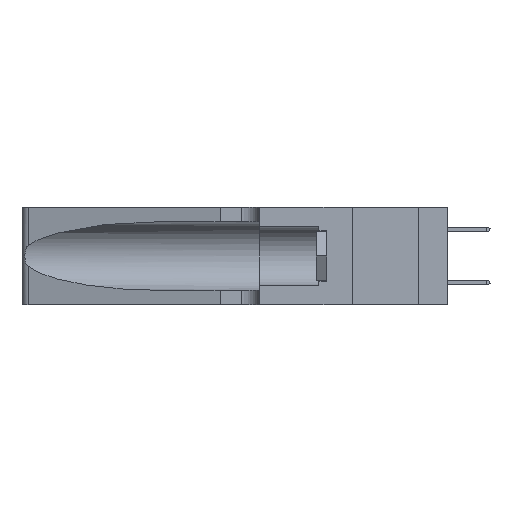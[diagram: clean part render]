
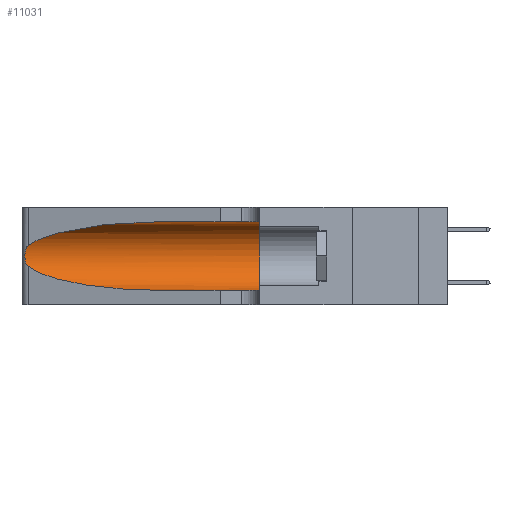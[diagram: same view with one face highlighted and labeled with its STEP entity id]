
A CAD part, left-side view. The second image highlights one B-rep face of the part: STEP entity #11031.
In plain terms, the highlighted cylindrical face has radius 3.308 mm (diameter 6.617 mm), a partial arc.
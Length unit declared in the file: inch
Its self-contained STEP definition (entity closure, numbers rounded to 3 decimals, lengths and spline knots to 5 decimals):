
#57 = CARTESIAN_POINT ( 'NONE',  ( 0.25487, 1.22718, 0.22369 ) ) ;
#100 = CARTESIAN_POINT ( 'NONE',  ( 0.1305, 0.72297, 0.31525 ) ) ;
#926 = CARTESIAN_POINT ( 'NONE',  ( 0.25487, 1.22718, 0.14631 ) ) ;
#1416 = EDGE_CURVE ( 'NONE', #9132, #16972, #7508, .T. ) ;
#1848 = CARTESIAN_POINT ( 'NONE',  ( 0.1305, 0.72297, 0.05475 ) ) ;
#1862 = ORIENTED_EDGE ( 'NONE', *, *, #10962, .T. ) ;
#2369 = CARTESIAN_POINT ( 'NONE',  ( 0.25487, 1.22718, 0.14631 ) ) ;
#2389 = CARTESIAN_POINT ( 'NONE',  ( 0.25639, 1.23184, 0.21858 ) ) ;
#2812 = ORIENTED_EDGE ( 'NONE', *, *, #8728, .F. ) ;
#2948 = CARTESIAN_POINT ( 'NONE',  ( 0.1305, 0.72297, 0.05475 ) ) ;
#3871 = CARTESIAN_POINT ( 'NONE',  ( 0.25854, 1.2359, 0.20912 ) ) ;
#4096 = EDGE_CURVE ( 'NONE', #6751, #18009, #15461, .T. ) ;
#4334 = LINE ( 'NONE', #5383, #11875 ) ;
#4336 = CARTESIAN_POINT ( 'NONE',  ( 0.2373, 1.15595, 0.08982 ) ) ;
#4714 = EDGE_CURVE ( 'NONE', #7164, #16972, #7858, .T. ) ;
#5213 = CARTESIAN_POINT ( 'NONE',  ( 0.1305, 0.72297, 0.31525 ) ) ;
#5281 = DIRECTION ( 'NONE',  ( 0., 1., 0. ) ) ;
#5329 = CARTESIAN_POINT ( 'NONE',  ( 0.26075, 1.23896, 0.19203 ) ) ;
#5383 = CARTESIAN_POINT ( 'NONE',  ( 0.1305, 1.61858, 0.31525 ) ) ;
#6339 = EDGE_CURVE ( 'NONE', #13664, #9132, #13586, .T. ) ;
#6751 = VERTEX_POINT ( 'NONE', #5213 ) ;
#6795 = CARTESIAN_POINT ( 'NONE',  ( 0.26017, 1.23833, 0.17102 ) ) ;
#7164 = VERTEX_POINT ( 'NONE', #17564 ) ;
#7508 = LINE ( 'NONE', #10287, #14470 ) ;
#7858 = CIRCLE ( 'NONE', #17360, 0.13025 ) ;
#8128 = CARTESIAN_POINT ( 'NONE',  ( 0.25555, 1.22994, 0.2215 ) ) ;
#8188 = CARTESIAN_POINT ( 'NONE',  ( 0.25789, 1.23486, 0.15765 ) ) ;
#8676 = CARTESIAN_POINT ( 'NONE',  ( 0.18966, 0.96281, 0.31525 ) ) ;
#8728 = EDGE_CURVE ( 'NONE', #6751, #7164, #4334, .T. ) ;
#9132 = VERTEX_POINT ( 'NONE', #1848 ) ;
#9367 = CARTESIAN_POINT ( 'NONE',  ( 0.25487, 1.22718, 0.22369 ) ) ;
#9573 = EDGE_LOOP ( 'NONE', ( #16071, #1862, #13246, #16939, #17371, #2812 ) ) ;
#9633 = CARTESIAN_POINT ( 'NONE',  ( 0.25555, 1.22993, 0.14849 ) ) ;
#9767 = DIRECTION ( 'NONE',  ( 0., -1., 0. ) ) ;
#10287 = CARTESIAN_POINT ( 'NONE',  ( 0.1305, 1.61858, 0.05475 ) ) ;
#10962 = EDGE_CURVE ( 'NONE', #18009, #13664, #14374, .T. ) ;
#11031 = ADVANCED_FACE ( 'NONE', ( #13854 ), #17135, .F. ) ;
#11493 = CARTESIAN_POINT ( 'NONE',  ( 0.25487, 1.22718, 0.14631 ) ) ;
#11875 = VECTOR ( 'NONE', #13809, 39.37008 ) ;
#12103 = CARTESIAN_POINT ( 'NONE',  ( 0.2373, 1.15595, 0.28018 ) ) ;
#12355 = CARTESIAN_POINT ( 'NONE',  ( 0.25787, 1.23484, 0.2124 ) ) ;
#13246 = ORIENTED_EDGE ( 'NONE', *, *, #6339, .T. ) ;
#13586 =( BOUNDED_CURVE ( )  B_SPLINE_CURVE ( 3, ( #11493, #4336, #17002, #2948 ),
 .UNSPECIFIED., .F., .T. ) 
 B_SPLINE_CURVE_WITH_KNOTS ( ( 4, 4 ),
 ( 3.44316, 4.71239 ),
 .UNSPECIFIED. ) 
 CURVE ( )  GEOMETRIC_REPRESENTATION_ITEM ( )  RATIONAL_B_SPLINE_CURVE ( ( 1., 0.87, 0.87, 1. ) ) 
 REPRESENTATION_ITEM ( '' )  );
#13664 = VERTEX_POINT ( 'NONE', #2369 ) ;
#13700 = CARTESIAN_POINT ( 'NONE',  ( 0.1305, 0.35, 0.185 ) ) ;
#13751 = CARTESIAN_POINT ( 'NONE',  ( 0.26018, 1.23835, 0.19895 ) ) ;
#13764 = CARTESIAN_POINT ( 'NONE',  ( 0.1305, 0.35, 0.05475 ) ) ;
#13809 = DIRECTION ( 'NONE',  ( 0., -1., 0. ) ) ;
#13854 = FACE_OUTER_BOUND ( 'NONE', #9573, .T. ) ;
#13865 = DIRECTION ( 'NONE',  ( 0., 0., -1. ) ) ;
#13954 = DIRECTION ( 'NONE',  ( 0., -1., 0. ) ) ;
#14374 = B_SPLINE_CURVE_WITH_KNOTS ( 'NONE', 3,
 ( #17854, #8128, #2389, #12355, #3871, #13751, #5329, #15123, #6795, #16553, #8188, #17911, #9633, #926 ),
 .UNSPECIFIED., .F., .F.,
 ( 4, 2, 2, 2, 2, 2, 4 ),
 ( 0., 0.00027, 0.00053, 0.00107, 0.0016, 0.00187, 0.00214 ),
 .UNSPECIFIED. ) ;
#14470 = VECTOR ( 'NONE', #13954, 39.37008 ) ;
#15075 = DIRECTION ( 'NONE',  ( 0., 0., 1. ) ) ;
#15123 = CARTESIAN_POINT ( 'NONE',  ( 0.26075, 1.23896, 0.178 ) ) ;
#15461 =( BOUNDED_CURVE ( )  B_SPLINE_CURVE ( 3, ( #100, #8676, #12103, #57 ),
 .UNSPECIFIED., .F., .F. ) 
 B_SPLINE_CURVE_WITH_KNOTS ( ( 4, 4 ),
 ( 1.5708, 2.84003 ),
 .UNSPECIFIED. ) 
 CURVE ( )  GEOMETRIC_REPRESENTATION_ITEM ( )  RATIONAL_B_SPLINE_CURVE ( ( 1., 0.87, 0.87, 1. ) ) 
 REPRESENTATION_ITEM ( '' )  );
#16071 = ORIENTED_EDGE ( 'NONE', *, *, #4096, .T. ) ;
#16367 = AXIS2_PLACEMENT_3D ( 'NONE', #16671, #9767, #13865 ) ;
#16553 = CARTESIAN_POINT ( 'NONE',  ( 0.25856, 1.23593, 0.16098 ) ) ;
#16671 = CARTESIAN_POINT ( 'NONE',  ( 0.1305, 1.61858, 0.185 ) ) ;
#16939 = ORIENTED_EDGE ( 'NONE', *, *, #1416, .T. ) ;
#16972 = VERTEX_POINT ( 'NONE', #13764 ) ;
#17002 = CARTESIAN_POINT ( 'NONE',  ( 0.18966, 0.96281, 0.05475 ) ) ;
#17135 = CYLINDRICAL_SURFACE ( 'NONE', #16367, 0.13025 ) ;
#17360 = AXIS2_PLACEMENT_3D ( 'NONE', #13700, #5281, #15075 ) ;
#17371 = ORIENTED_EDGE ( 'NONE', *, *, #4714, .F. ) ;
#17564 = CARTESIAN_POINT ( 'NONE',  ( 0.1305, 0.35, 0.31525 ) ) ;
#17854 = CARTESIAN_POINT ( 'NONE',  ( 0.25487, 1.22718, 0.22369 ) ) ;
#17911 = CARTESIAN_POINT ( 'NONE',  ( 0.25639, 1.23186, 0.15144 ) ) ;
#18009 = VERTEX_POINT ( 'NONE', #9367 ) ;
